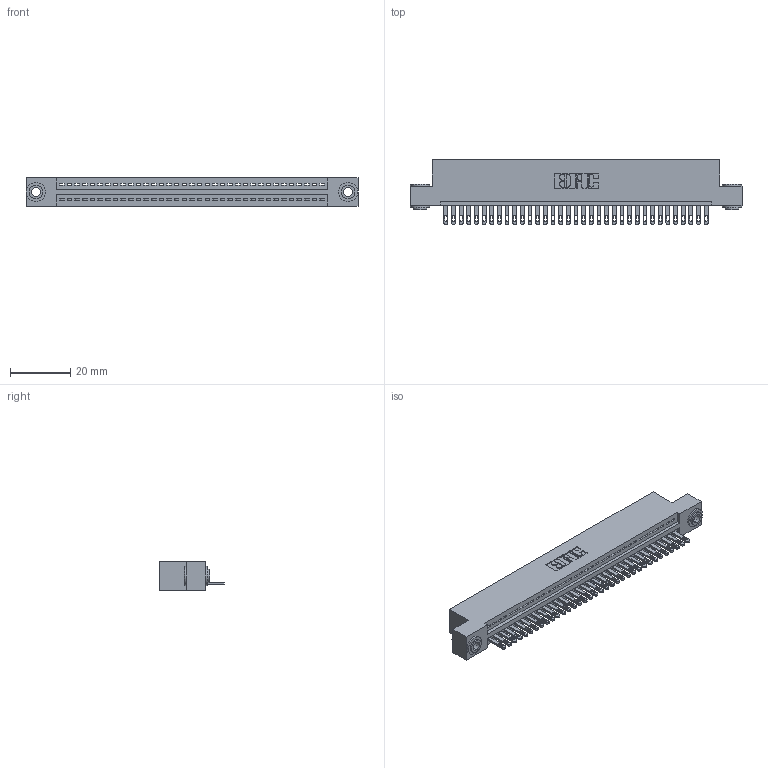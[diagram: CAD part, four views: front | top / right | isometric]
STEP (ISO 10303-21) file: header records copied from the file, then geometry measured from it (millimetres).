
FILE_DESCRIPTION (( 'STEP AP203' ), '1' );
FILE_NAME ('895-035-500-103.STEP', '2020-09-25T22:11:25', ( '' ), ( '' ), 'SwSTEP 2.0', 'SolidWorks 2020', '' );
FILE_SCHEMA (( 'CONFIG_CONTROL_DESIGN' ));
Length unit declared in the file: inch
Products named in the file (4): 345-292-001_345-293-100; 345-250-002_345-250-002-102; 895-035-500-103; 845 Part_Flush Mounting Lugs - 0.156 Dia-TH
Assembly tree (38 placements, depth 2):
  895-035-500-103
    845 Part_Flush Mounting Lugs - 0.156 Dia-TH
    345-292-001_345-293-100  x35
    345-250-002_345-250-002-102  x2
Bounding box: 110.11 x 21.51 x 9.4 mm (x, y, z)
Volume: 10442 mm3; surface area: 14074.4 mm2
Topology: 38 solids, 38 shells, 2054 faces, 6297 edges, 4194 vertices
Faces by surface type: plane 1280, cylinder 766, cone 8
Entity records: 27864 total; most frequent: CARTESIAN_POINT 4804, ORIENTED_EDGE 4766, DIRECTION 4239, EDGE_CURVE 2383, VECTOR 2083, LINE 2083, VERTEX_POINT 1586, AXIS2_PLACEMENT_3D 1078
